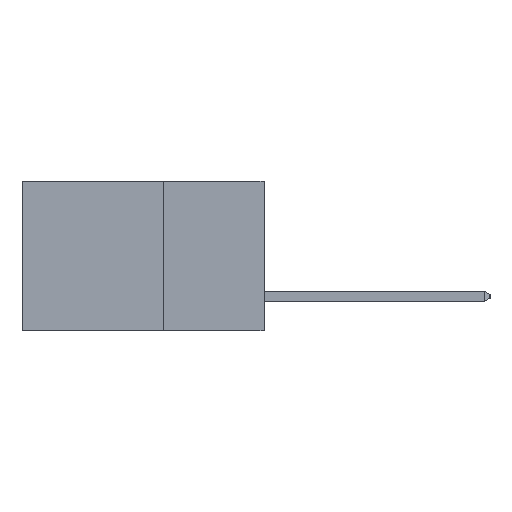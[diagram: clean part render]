
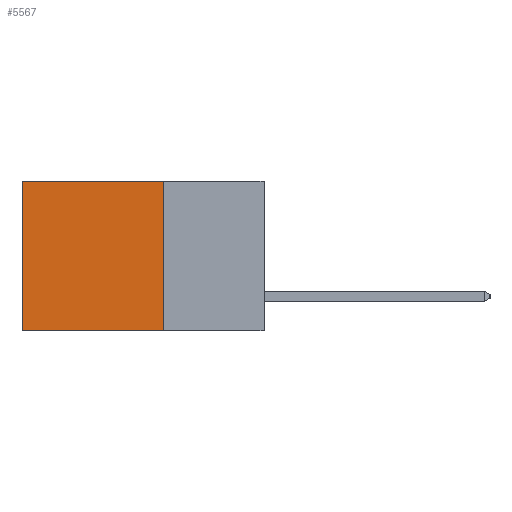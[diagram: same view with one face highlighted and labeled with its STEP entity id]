
A CAD part, left-side view. The second image highlights one B-rep face of the part: STEP entity #5567.
In plain terms, the highlighted planar face has unit normal (-1, 0, 0).
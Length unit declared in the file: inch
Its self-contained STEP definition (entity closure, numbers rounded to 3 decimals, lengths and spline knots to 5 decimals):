
#1171 = VERTEX_POINT ( 'NONE', #4539 ) ;
#1304 = CARTESIAN_POINT ( 'NONE',  ( 0.2615, 0.6, -0.37 ) ) ;
#2803 = CARTESIAN_POINT ( 'NONE',  ( 0.2615, 0.6, -0.37 ) ) ;
#3397 = FACE_OUTER_BOUND ( 'NONE', #7486, .T. ) ;
#3745 = VECTOR ( 'NONE', #5343, 39.37008 ) ;
#3832 = VECTOR ( 'NONE', #8325, 39.37008 ) ;
#4236 = CARTESIAN_POINT ( 'NONE',  ( 0.2615, 0.25, -0.37 ) ) ;
#4539 = CARTESIAN_POINT ( 'NONE',  ( 0.2615, 0.25, 0. ) ) ;
#4854 = DIRECTION ( 'NONE',  ( 0., 0., -1. ) ) ;
#5135 = ORIENTED_EDGE ( 'NONE', *, *, #11051, .T. ) ;
#5343 = DIRECTION ( 'NONE',  ( 0., 1., 0. ) ) ;
#5565 = EDGE_CURVE ( 'NONE', #8042, #6526, #6377, .T. ) ;
#5567 = ADVANCED_FACE ( 'NONE', ( #3397 ), #11955, .F. ) ;
#5622 = ORIENTED_EDGE ( 'NONE', *, *, #10491, .T. ) ;
#5982 = CARTESIAN_POINT ( 'NONE',  ( 0.2615, 0.25, -0.37 ) ) ;
#6377 = LINE ( 'NONE', #4236, #3745 ) ;
#6526 = VERTEX_POINT ( 'NONE', #1304 ) ;
#7008 = ORIENTED_EDGE ( 'NONE', *, *, #11775, .F. ) ;
#7216 = CARTESIAN_POINT ( 'NONE',  ( 0.2615, 0.25, 0. ) ) ;
#7486 = EDGE_LOOP ( 'NONE', ( #5622, #13106, #7008, #5135 ) ) ;
#7588 = DIRECTION ( 'NONE',  ( 0., 0., -1. ) ) ;
#8023 = LINE ( 'NONE', #2803, #13832 ) ;
#8042 = VERTEX_POINT ( 'NONE', #13927 ) ;
#8325 = DIRECTION ( 'NONE',  ( 0., 1., 0. ) ) ;
#8899 = VECTOR ( 'NONE', #4854, 39.37008 ) ;
#8996 = AXIS2_PLACEMENT_3D ( 'NONE', #13053, #14124, #7588 ) ;
#9321 = VERTEX_POINT ( 'NONE', #10640 ) ;
#10491 = EDGE_CURVE ( 'NONE', #9321, #6526, #8023, .T. ) ;
#10610 = DIRECTION ( 'NONE',  ( 0., 0., -1. ) ) ;
#10640 = CARTESIAN_POINT ( 'NONE',  ( 0.2615, 0.6, 0. ) ) ;
#11051 = EDGE_CURVE ( 'NONE', #1171, #9321, #12666, .T. ) ;
#11775 = EDGE_CURVE ( 'NONE', #1171, #8042, #12131, .T. ) ;
#11955 = PLANE ( 'NONE',  #8996 ) ;
#12131 = LINE ( 'NONE', #5982, #8899 ) ;
#12666 = LINE ( 'NONE', #7216, #3832 ) ;
#13053 = CARTESIAN_POINT ( 'NONE',  ( 0.2615, 0.25, -0.37 ) ) ;
#13106 = ORIENTED_EDGE ( 'NONE', *, *, #5565, .F. ) ;
#13832 = VECTOR ( 'NONE', #10610, 39.37008 ) ;
#13927 = CARTESIAN_POINT ( 'NONE',  ( 0.2615, 0.25, -0.37 ) ) ;
#14124 = DIRECTION ( 'NONE',  ( 1., 0., 0. ) ) ;
